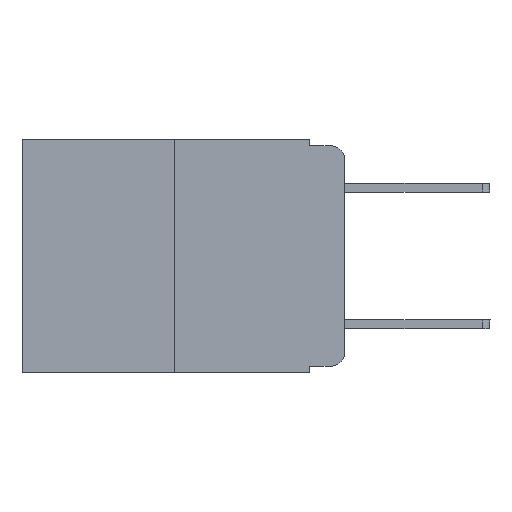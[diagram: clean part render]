
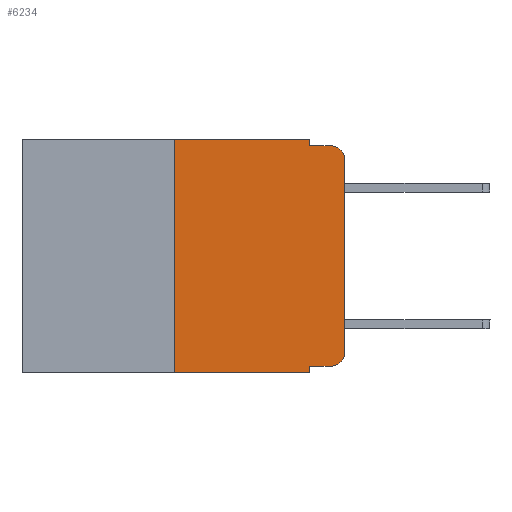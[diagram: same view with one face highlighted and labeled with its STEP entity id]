
A CAD part, left-side view. The second image highlights one B-rep face of the part: STEP entity #6234.
In plain terms, the highlighted planar face has unit normal (-1, 0, 0).
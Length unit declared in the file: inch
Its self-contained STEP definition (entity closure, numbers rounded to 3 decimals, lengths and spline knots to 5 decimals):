
#287 = ORIENTED_EDGE ( 'NONE', *, *, #10329, .T. ) ;
#520 = CARTESIAN_POINT ( 'NONE',  ( 0., 0.25, -0.343 ) ) ;
#638 = EDGE_LOOP ( 'NONE', ( #13529, #14469, #9539, #10237, #8742, #5825, #10297, #2811, #287, #3108 ) ) ;
#728 = CARTESIAN_POINT ( 'NONE',  ( 0., 0.051, -0.01 ) ) ;
#944 = LINE ( 'NONE', #3500, #13190 ) ;
#1214 = DIRECTION ( 'NONE',  ( 0., 0., 1. ) ) ;
#1605 = VERTEX_POINT ( 'NONE', #5823 ) ;
#2052 = EDGE_CURVE ( 'NONE', #1605, #4023, #13193, .T. ) ;
#2618 = CARTESIAN_POINT ( 'NONE',  ( 0., 0.25, 0. ) ) ;
#2732 = LINE ( 'NONE', #13976, #15178 ) ;
#2811 = ORIENTED_EDGE ( 'NONE', *, *, #13677, .F. ) ;
#2959 = DIRECTION ( 'NONE',  ( 0., 0., -1. ) ) ;
#3048 = VERTEX_POINT ( 'NONE', #5496 ) ;
#3108 = ORIENTED_EDGE ( 'NONE', *, *, #13406, .T. ) ;
#3500 = CARTESIAN_POINT ( 'NONE',  ( 0., 0.051, -0.333 ) ) ;
#3530 = AXIS2_PLACEMENT_3D ( 'NONE', #9286, #7106, #6868 ) ;
#3622 = VECTOR ( 'NONE', #4418, 39.37008 ) ;
#4023 = VERTEX_POINT ( 'NONE', #6657 ) ;
#4100 = PLANE ( 'NONE',  #14038 ) ;
#4210 = LINE ( 'NONE', #11224, #15791 ) ;
#4331 = LINE ( 'NONE', #728, #3622 ) ;
#4345 = VERTEX_POINT ( 'NONE', #520 ) ;
#4418 = DIRECTION ( 'NONE',  ( 0., -1., 0. ) ) ;
#4431 = DIRECTION ( 'NONE',  ( 0., 0., -1. ) ) ;
#5348 = EDGE_CURVE ( 'NONE', #4023, #8872, #14814, .T. ) ;
#5496 = CARTESIAN_POINT ( 'NONE',  ( 0., 0.051, -0.01 ) ) ;
#5560 = CARTESIAN_POINT ( 'NONE',  ( 0., 0.051, -0.333 ) ) ;
#5598 = VERTEX_POINT ( 'NONE', #2618 ) ;
#5649 = DIRECTION ( 'NONE',  ( 0., -1., 0. ) ) ;
#5823 = CARTESIAN_POINT ( 'NONE',  ( 0., 0., -0.313 ) ) ;
#5825 = ORIENTED_EDGE ( 'NONE', *, *, #10926, .F. ) ;
#6234 = ADVANCED_FACE ( 'NONE', ( #15111 ), #4100, .F. ) ;
#6657 = CARTESIAN_POINT ( 'NONE',  ( 0., 0., -0.03 ) ) ;
#6786 = DIRECTION ( 'NONE',  ( 0., -1., 0. ) ) ;
#6868 = DIRECTION ( 'NONE',  ( 0., 0., -1. ) ) ;
#7106 = DIRECTION ( 'NONE',  ( -1., 0., 0. ) ) ;
#7149 = EDGE_CURVE ( 'NONE', #5598, #8871, #15540, .T. ) ;
#7955 = CARTESIAN_POINT ( 'NONE',  ( 0., 0.02, -0.01 ) ) ;
#8020 = VECTOR ( 'NONE', #5649, 39.37008 ) ;
#8363 = EDGE_CURVE ( 'NONE', #4345, #13238, #4210, .T. ) ;
#8742 = ORIENTED_EDGE ( 'NONE', *, *, #7149, .F. ) ;
#8871 = VERTEX_POINT ( 'NONE', #11572 ) ;
#8872 = VERTEX_POINT ( 'NONE', #7955 ) ;
#9037 = VERTEX_POINT ( 'NONE', #15674 ) ;
#9266 = CARTESIAN_POINT ( 'NONE',  ( 0., 0.473, 0. ) ) ;
#9286 = CARTESIAN_POINT ( 'NONE',  ( 0., 0.02, -0.03 ) ) ;
#9539 = ORIENTED_EDGE ( 'NONE', *, *, #14952, .F. ) ;
#9606 = DIRECTION ( 'NONE',  ( 0., -1., 0. ) ) ;
#9621 = DIRECTION ( 'NONE',  ( 1., 0., 0. ) ) ;
#9726 = CARTESIAN_POINT ( 'NONE',  ( 0., 0., 0. ) ) ;
#10237 = ORIENTED_EDGE ( 'NONE', *, *, #15230, .F. ) ;
#10297 = ORIENTED_EDGE ( 'NONE', *, *, #8363, .T. ) ;
#10329 = EDGE_CURVE ( 'NONE', #11136, #9037, #944, .T. ) ;
#10639 = CARTESIAN_POINT ( 'NONE',  ( 0., 0.02, -0.313 ) ) ;
#10926 = EDGE_CURVE ( 'NONE', #4345, #5598, #11350, .T. ) ;
#11082 = CARTESIAN_POINT ( 'NONE',  ( 0., 0.051, -0.343 ) ) ;
#11136 = VERTEX_POINT ( 'NONE', #5560 ) ;
#11224 = CARTESIAN_POINT ( 'NONE',  ( 0., 0.473, -0.343 ) ) ;
#11350 = LINE ( 'NONE', #12225, #12521 ) ;
#11572 = CARTESIAN_POINT ( 'NONE',  ( 0., 0.051, 0. ) ) ;
#12225 = CARTESIAN_POINT ( 'NONE',  ( 0., 0.25, 0. ) ) ;
#12329 = VECTOR ( 'NONE', #1214, 39.37008 ) ;
#12521 = VECTOR ( 'NONE', #14887, 39.37008 ) ;
#12550 = AXIS2_PLACEMENT_3D ( 'NONE', #10639, #12593, #14342 ) ;
#12593 = DIRECTION ( 'NONE',  ( -1., 0., 0. ) ) ;
#13190 = VECTOR ( 'NONE', #9606, 39.37008 ) ;
#13193 = LINE ( 'NONE', #9726, #12329 ) ;
#13238 = VERTEX_POINT ( 'NONE', #11082 ) ;
#13406 = EDGE_CURVE ( 'NONE', #9037, #1605, #14656, .T. ) ;
#13529 = ORIENTED_EDGE ( 'NONE', *, *, #2052, .T. ) ;
#13677 = EDGE_CURVE ( 'NONE', #11136, #13238, #15438, .T. ) ;
#13976 = CARTESIAN_POINT ( 'NONE',  ( 0., 0.051, 0. ) ) ;
#14038 = AXIS2_PLACEMENT_3D ( 'NONE', #14061, #9621, #15276 ) ;
#14061 = CARTESIAN_POINT ( 'NONE',  ( 0., 0.473, 0. ) ) ;
#14315 = CARTESIAN_POINT ( 'NONE',  ( 0., 0.051, 0. ) ) ;
#14342 = DIRECTION ( 'NONE',  ( 0., 0., -1. ) ) ;
#14469 = ORIENTED_EDGE ( 'NONE', *, *, #5348, .T. ) ;
#14656 = CIRCLE ( 'NONE', #12550, 0.02 ) ;
#14814 = CIRCLE ( 'NONE', #3530, 0.02 ) ;
#14887 = DIRECTION ( 'NONE',  ( 0., 0., 1. ) ) ;
#14952 = EDGE_CURVE ( 'NONE', #3048, #8872, #4331, .T. ) ;
#15111 = FACE_OUTER_BOUND ( 'NONE', #638, .T. ) ;
#15142 = VECTOR ( 'NONE', #4431, 39.37008 ) ;
#15178 = VECTOR ( 'NONE', #2959, 39.37008 ) ;
#15230 = EDGE_CURVE ( 'NONE', #8871, #3048, #2732, .T. ) ;
#15276 = DIRECTION ( 'NONE',  ( 0., 0., -1. ) ) ;
#15438 = LINE ( 'NONE', #14315, #15142 ) ;
#15540 = LINE ( 'NONE', #9266, #8020 ) ;
#15674 = CARTESIAN_POINT ( 'NONE',  ( 0., 0.02, -0.333 ) ) ;
#15791 = VECTOR ( 'NONE', #6786, 39.37008 ) ;
